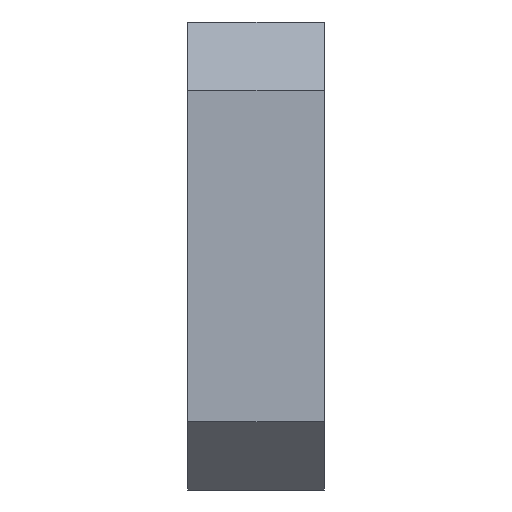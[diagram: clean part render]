
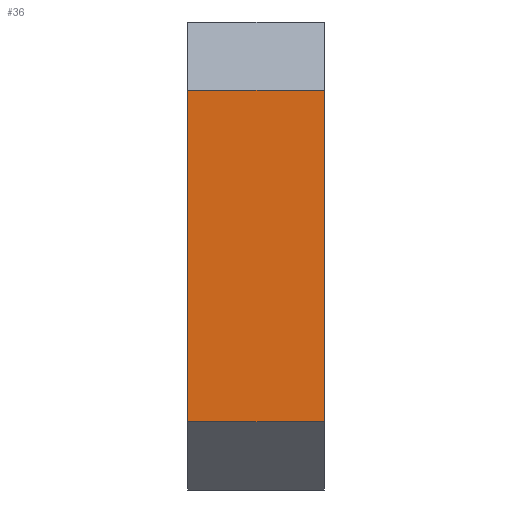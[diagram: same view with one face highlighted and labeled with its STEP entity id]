
A CAD part, left-side view. The second image highlights one B-rep face of the part: STEP entity #36.
In plain terms, the highlighted planar face has unit normal (-1, 0, 0).
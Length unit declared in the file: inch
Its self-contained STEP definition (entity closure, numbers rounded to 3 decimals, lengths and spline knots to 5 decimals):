
#34 = VERTEX_POINT ( 'NONE', #519 ) ;
#36 = ADVANCED_FACE ( 'NONE', ( #285 ), #462, .F. ) ;
#47 = VERTEX_POINT ( 'NONE', #418 ) ;
#76 = VECTOR ( 'NONE', #520, 39.37008 ) ;
#94 = ORIENTED_EDGE ( 'NONE', *, *, #349, .T. ) ;
#114 = LINE ( 'NONE', #547, #487 ) ;
#144 = ORIENTED_EDGE ( 'NONE', *, *, #265, .F. ) ;
#155 = ORIENTED_EDGE ( 'NONE', *, *, #354, .F. ) ;
#156 = CARTESIAN_POINT ( 'NONE',  ( -1.069, 0., 0.1525 ) ) ;
#166 = VERTEX_POINT ( 'NONE', #156 ) ;
#167 = ORIENTED_EDGE ( 'NONE', *, *, #341, .T. ) ;
#169 = AXIS2_PLACEMENT_3D ( 'NONE', #503, #477, #475 ) ;
#172 = DIRECTION ( 'NONE',  ( 0., 1., 0. ) ) ;
#216 = CARTESIAN_POINT ( 'NONE',  ( -1.069, -0.125, -0.1525 ) ) ;
#239 = LINE ( 'NONE', #561, #76 ) ;
#265 = EDGE_CURVE ( 'NONE', #34, #387, #623, .T. ) ;
#285 = FACE_OUTER_BOUND ( 'NONE', #645, .T. ) ;
#341 = EDGE_CURVE ( 'NONE', #47, #166, #497, .T. ) ;
#349 = EDGE_CURVE ( 'NONE', #166, #387, #114, .T. ) ;
#354 = EDGE_CURVE ( 'NONE', #47, #34, #239, .T. ) ;
#387 = VERTEX_POINT ( 'NONE', #402 ) ;
#402 = CARTESIAN_POINT ( 'NONE',  ( -1.069, 0., -0.1525 ) ) ;
#405 = VECTOR ( 'NONE', #589, 39.37008 ) ;
#418 = CARTESIAN_POINT ( 'NONE',  ( -1.069, -0.125, 0.1525 ) ) ;
#462 = PLANE ( 'NONE',  #169 ) ;
#475 = DIRECTION ( 'NONE',  ( 0., 0., -1. ) ) ;
#477 = DIRECTION ( 'NONE',  ( 1., 0., 0. ) ) ;
#487 = VECTOR ( 'NONE', #529, 39.37008 ) ;
#497 = LINE ( 'NONE', #583, #405 ) ;
#503 = CARTESIAN_POINT ( 'NONE',  ( -1.069, -0.125, 0.1525 ) ) ;
#519 = CARTESIAN_POINT ( 'NONE',  ( -1.069, -0.125, -0.1525 ) ) ;
#520 = DIRECTION ( 'NONE',  ( 0., 0., -1. ) ) ;
#525 = VECTOR ( 'NONE', #172, 39.37008 ) ;
#529 = DIRECTION ( 'NONE',  ( 0., 0., -1. ) ) ;
#547 = CARTESIAN_POINT ( 'NONE',  ( -1.069, 0., 0.1525 ) ) ;
#561 = CARTESIAN_POINT ( 'NONE',  ( -1.069, -0.125, 0.1525 ) ) ;
#583 = CARTESIAN_POINT ( 'NONE',  ( -1.069, -0.125, 0.1525 ) ) ;
#589 = DIRECTION ( 'NONE',  ( 0., 1., 0. ) ) ;
#623 = LINE ( 'NONE', #216, #525 ) ;
#645 = EDGE_LOOP ( 'NONE', ( #94, #144, #155, #167 ) ) ;
